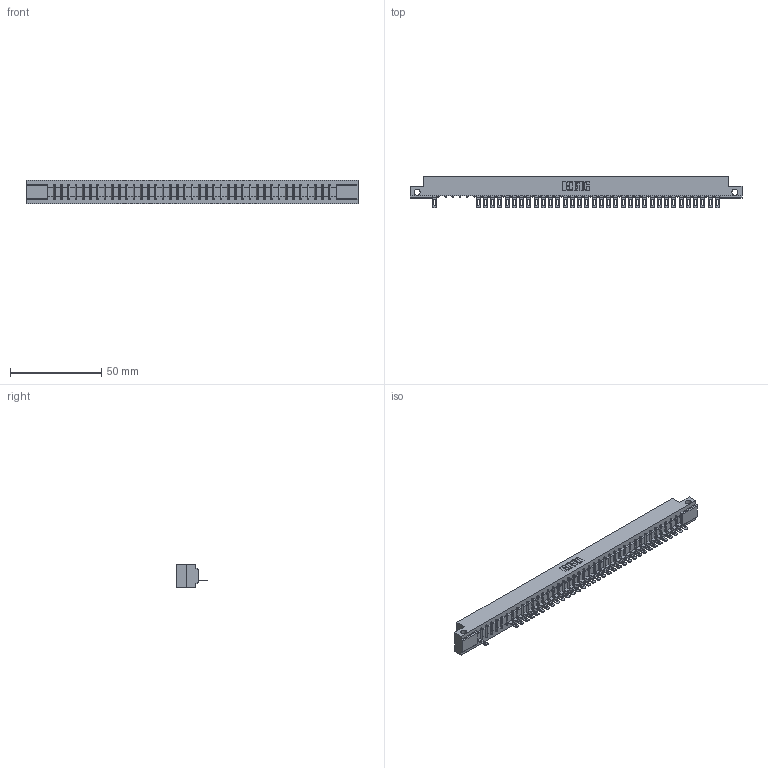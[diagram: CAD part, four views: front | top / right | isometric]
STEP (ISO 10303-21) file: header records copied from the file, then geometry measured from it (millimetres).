
FILE_DESCRIPTION (( 'STEP AP203' ), '1' );
FILE_NAME ('357-040-501-112.STEP', '2018-08-11T05:15:23', ( '' ), ( '' ), 'SwSTEP 2.0', 'SolidWorks 2016', '' );
FILE_SCHEMA (( 'CONFIG_CONTROL_DESIGN' ));
Length unit declared in the file: inch
Products named in the file (3): 307 Part_.128 Dia Side Mounting Holes; 307-290-002_501; 357-040-501-112
Assembly tree (36 placements, depth 2):
  357-040-501-112
    307 Part_.128 Dia Side Mounting Holes
    307-290-002_501  x35
Bounding box: 181.51 x 17.42 x 12.7 mm (x, y, z)
Volume: 19152.5 mm3; surface area: 23336.4 mm2
Topology: 36 solids, 36 shells, 2919 faces, 8973 edges, 5870 vertices
Faces by surface type: plane 1670, cylinder 1167, sphere 82
Entity records: 35174 total; most frequent: CARTESIAN_POINT 5955, ORIENTED_EDGE 5950, DIRECTION 5785, EDGE_CURVE 2975, LINE 2273, VECTOR 2273, VERTEX_POINT 1926, AXIS2_PLACEMENT_3D 1756
